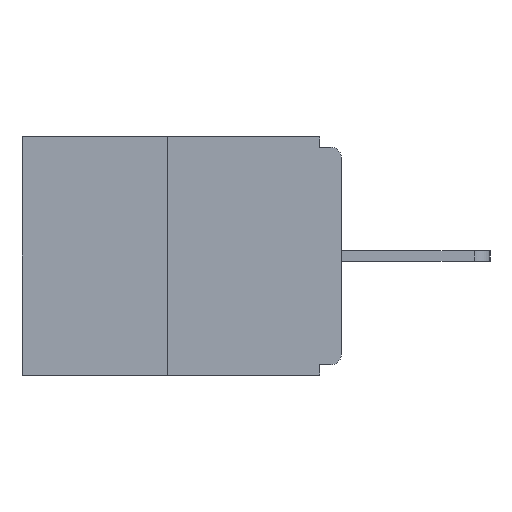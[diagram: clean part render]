
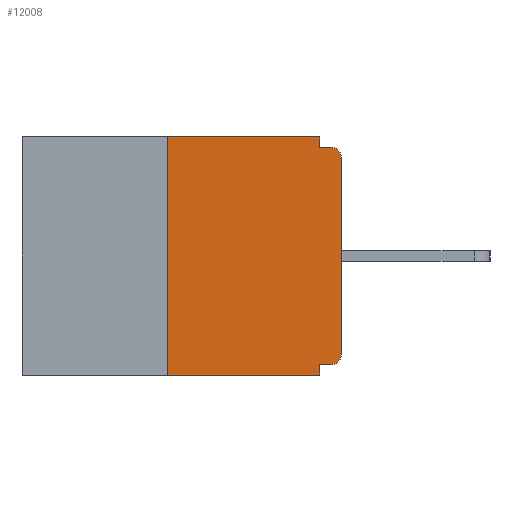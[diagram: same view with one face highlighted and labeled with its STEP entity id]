
A CAD part, left-side view. The second image highlights one B-rep face of the part: STEP entity #12008.
In plain terms, the highlighted planar face has unit normal (-1, 0, 0).
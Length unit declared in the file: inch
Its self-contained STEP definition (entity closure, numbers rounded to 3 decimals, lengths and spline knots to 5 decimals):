
#364 = VERTEX_POINT ( 'NONE', #11985 ) ;
#435 = VERTEX_POINT ( 'NONE', #16937 ) ;
#465 = DIRECTION ( 'NONE',  ( 0., 0., -1. ) ) ;
#512 = CARTESIAN_POINT ( 'NONE',  ( 0., 0., -0.015 ) ) ;
#914 = CARTESIAN_POINT ( 'NONE',  ( 0., 0.031, -0.343 ) ) ;
#1598 = DIRECTION ( 'NONE',  ( 0., 0., -1. ) ) ;
#1723 = CARTESIAN_POINT ( 'NONE',  ( 0., 0.031, 0. ) ) ;
#1964 = CARTESIAN_POINT ( 'NONE',  ( 0., 0.46, 0. ) ) ;
#2328 = CARTESIAN_POINT ( 'NONE',  ( 0., 0.46, -0.343 ) ) ;
#2342 = CARTESIAN_POINT ( 'NONE',  ( 0., 0.015, -0.313 ) ) ;
#2418 = ORIENTED_EDGE ( 'NONE', *, *, #14739, .F. ) ;
#2478 = FACE_OUTER_BOUND ( 'NONE', #16299, .T. ) ;
#2709 = VECTOR ( 'NONE', #3308, 39.37008 ) ;
#3308 = DIRECTION ( 'NONE',  ( 0., 1., 0. ) ) ;
#3418 = AXIS2_PLACEMENT_3D ( 'NONE', #1964, #22296, #18207 ) ;
#3483 = VERTEX_POINT ( 'NONE', #10432 ) ;
#3589 = LINE ( 'NONE', #1723, #18781 ) ;
#4281 = CIRCLE ( 'NONE', #24605, 0.015 ) ;
#4387 = LINE ( 'NONE', #12491, #5882 ) ;
#4435 = VERTEX_POINT ( 'NONE', #914 ) ;
#4503 = VERTEX_POINT ( 'NONE', #10213 ) ;
#4586 = VERTEX_POINT ( 'NONE', #10195 ) ;
#5025 = VECTOR ( 'NONE', #20598, 39.37008 ) ;
#5882 = VECTOR ( 'NONE', #10633, 39.37008 ) ;
#6953 = EDGE_CURVE ( 'NONE', #14605, #4586, #3589, .T. ) ;
#8068 = CIRCLE ( 'NONE', #12335, 0.015 ) ;
#8138 = EDGE_CURVE ( 'NONE', #364, #435, #23642, .T. ) ;
#8711 = EDGE_CURVE ( 'NONE', #9069, #24984, #4281, .T. ) ;
#9069 = VERTEX_POINT ( 'NONE', #17812 ) ;
#9473 = CARTESIAN_POINT ( 'NONE',  ( 0., 0.015, -0.03 ) ) ;
#9532 = VECTOR ( 'NONE', #465, 39.37008 ) ;
#10195 = CARTESIAN_POINT ( 'NONE',  ( 0., 0.031, -0.015 ) ) ;
#10213 = CARTESIAN_POINT ( 'NONE',  ( 0., 0.25, -0.343 ) ) ;
#10261 = EDGE_CURVE ( 'NONE', #4586, #24984, #14499, .T. ) ;
#10323 = EDGE_CURVE ( 'NONE', #17366, #9069, #4387, .T. ) ;
#10432 = CARTESIAN_POINT ( 'NONE',  ( 0., 0.25, 0. ) ) ;
#10633 = DIRECTION ( 'NONE',  ( 0., 0., 1. ) ) ;
#11668 = VECTOR ( 'NONE', #18436, 39.37008 ) ;
#11985 = CARTESIAN_POINT ( 'NONE',  ( 0., 0.015, -0.328 ) ) ;
#12008 = ADVANCED_FACE ( 'NONE', ( #2478 ), #12463, .F. ) ;
#12026 = EDGE_CURVE ( 'NONE', #364, #17366, #8068, .T. ) ;
#12188 = LINE ( 'NONE', #22157, #9532 ) ;
#12335 = AXIS2_PLACEMENT_3D ( 'NONE', #2342, #24269, #18712 ) ;
#12463 = PLANE ( 'NONE',  #3418 ) ;
#12491 = CARTESIAN_POINT ( 'NONE',  ( 0., 0., 0. ) ) ;
#12700 = ORIENTED_EDGE ( 'NONE', *, *, #8711, .T. ) ;
#13169 = CARTESIAN_POINT ( 'NONE',  ( 0., 0.25, 0. ) ) ;
#14256 = DIRECTION ( 'NONE',  ( 0., -1., 0. ) ) ;
#14499 = LINE ( 'NONE', #512, #5025 ) ;
#14605 = VERTEX_POINT ( 'NONE', #15934 ) ;
#14733 = EDGE_CURVE ( 'NONE', #4503, #4435, #16456, .T. ) ;
#14739 = EDGE_CURVE ( 'NONE', #435, #4435, #12188, .T. ) ;
#14929 = ORIENTED_EDGE ( 'NONE', *, *, #12026, .T. ) ;
#14943 = ORIENTED_EDGE ( 'NONE', *, *, #10261, .F. ) ;
#15934 = CARTESIAN_POINT ( 'NONE',  ( 0., 0.031, 0. ) ) ;
#16003 = DIRECTION ( 'NONE',  ( 0., 0., -1. ) ) ;
#16299 = EDGE_LOOP ( 'NONE', ( #20272, #19075, #22621, #2418, #25175, #14929, #25505, #12700, #14943, #19781 ) ) ;
#16456 = LINE ( 'NONE', #2328, #11668 ) ;
#16937 = CARTESIAN_POINT ( 'NONE',  ( 0., 0.031, -0.328 ) ) ;
#17366 = VERTEX_POINT ( 'NONE', #17554 ) ;
#17474 = EDGE_CURVE ( 'NONE', #4503, #3483, #23511, .T. ) ;
#17554 = CARTESIAN_POINT ( 'NONE',  ( 0., 0., -0.313 ) ) ;
#17812 = CARTESIAN_POINT ( 'NONE',  ( 0., 0., -0.03 ) ) ;
#18207 = DIRECTION ( 'NONE',  ( 0., 0., -1. ) ) ;
#18436 = DIRECTION ( 'NONE',  ( 0., -1., 0. ) ) ;
#18498 = LINE ( 'NONE', #22341, #19843 ) ;
#18712 = DIRECTION ( 'NONE',  ( 0., 0., -1. ) ) ;
#18779 = CARTESIAN_POINT ( 'NONE',  ( 0., 0.015, -0.015 ) ) ;
#18781 = VECTOR ( 'NONE', #1598, 39.37008 ) ;
#19002 = EDGE_CURVE ( 'NONE', #3483, #14605, #18498, .T. ) ;
#19075 = ORIENTED_EDGE ( 'NONE', *, *, #17474, .F. ) ;
#19537 = CARTESIAN_POINT ( 'NONE',  ( 0., 0., -0.328 ) ) ;
#19781 = ORIENTED_EDGE ( 'NONE', *, *, #6953, .F. ) ;
#19843 = VECTOR ( 'NONE', #14256, 39.37008 ) ;
#20272 = ORIENTED_EDGE ( 'NONE', *, *, #19002, .F. ) ;
#20598 = DIRECTION ( 'NONE',  ( 0., -1., 0. ) ) ;
#21656 = DIRECTION ( 'NONE',  ( 0., 0., 1. ) ) ;
#22157 = CARTESIAN_POINT ( 'NONE',  ( 0., 0.031, -0.343 ) ) ;
#22296 = DIRECTION ( 'NONE',  ( 1., 0., 0. ) ) ;
#22341 = CARTESIAN_POINT ( 'NONE',  ( 0., 0.46, 0. ) ) ;
#22621 = ORIENTED_EDGE ( 'NONE', *, *, #14733, .T. ) ;
#23511 = LINE ( 'NONE', #13169, #24474 ) ;
#23642 = LINE ( 'NONE', #19537, #2709 ) ;
#24269 = DIRECTION ( 'NONE',  ( -1., 0., 0. ) ) ;
#24474 = VECTOR ( 'NONE', #21656, 39.37008 ) ;
#24605 = AXIS2_PLACEMENT_3D ( 'NONE', #9473, #26083, #16003 ) ;
#24984 = VERTEX_POINT ( 'NONE', #18779 ) ;
#25175 = ORIENTED_EDGE ( 'NONE', *, *, #8138, .F. ) ;
#25505 = ORIENTED_EDGE ( 'NONE', *, *, #10323, .T. ) ;
#26083 = DIRECTION ( 'NONE',  ( -1., 0., 0. ) ) ;
